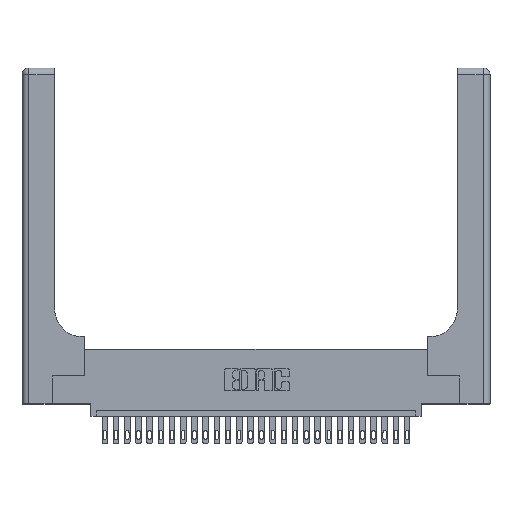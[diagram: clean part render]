
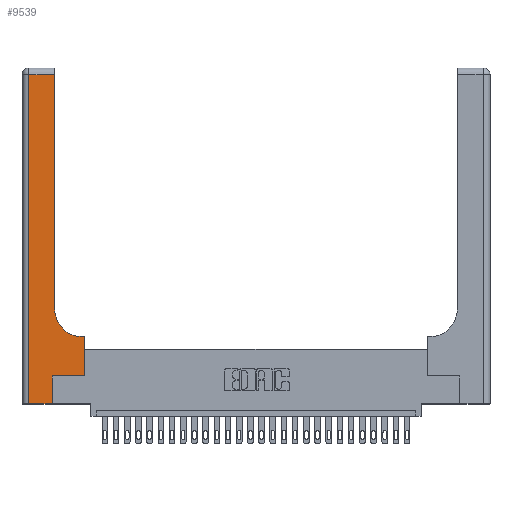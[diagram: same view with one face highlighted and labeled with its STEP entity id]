
A CAD part, top view. The second image highlights one B-rep face of the part: STEP entity #9539.
In plain terms, the highlighted planar face has unit normal (0, 0, 1).
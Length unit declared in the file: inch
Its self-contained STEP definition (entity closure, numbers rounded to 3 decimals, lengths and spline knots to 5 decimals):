
#55 = AXIS2_PLACEMENT_3D ( 'NONE', #7930, #12382, #5728 ) ;
#1465 = LINE ( 'NONE', #8245, #6556 ) ;
#1484 = EDGE_CURVE ( 'NONE', #8005, #10899, #6415, .T. ) ;
#1764 = DIRECTION ( 'NONE',  ( 0., -1., 0. ) ) ;
#2277 = DIRECTION ( 'NONE',  ( 0., 0., -1. ) ) ;
#3177 = DIRECTION ( 'NONE',  ( 0., 1., 0. ) ) ;
#3617 = EDGE_CURVE ( 'NONE', #11968, #6783, #13105, .T. ) ;
#3693 = DIRECTION ( 'NONE',  ( 0., 1., 0. ) ) ;
#3818 = DIRECTION ( 'NONE',  ( 1., 0., 0. ) ) ;
#4117 = EDGE_CURVE ( 'NONE', #6783, #14151, #5248, .T. ) ;
#4333 = VERTEX_POINT ( 'NONE', #11165 ) ;
#4653 = CARTESIAN_POINT ( 'NONE',  ( 0.269, 0., 0.37 ) ) ;
#5010 = EDGE_CURVE ( 'NONE', #26313, #11968, #1465, .T. ) ;
#5248 = LINE ( 'NONE', #4653, #22230 ) ;
#5728 = DIRECTION ( 'NONE',  ( -1., 0., 0. ) ) ;
#6003 = CARTESIAN_POINT ( 'NONE',  ( 0., 0., 0.37 ) ) ;
#6194 = EDGE_CURVE ( 'NONE', #14151, #4333, #14451, .T. ) ;
#6415 = CIRCLE ( 'NONE', #10715, 0.25 ) ;
#6529 = EDGE_CURVE ( 'NONE', #4333, #27735, #20626, .T. ) ;
#6556 = VECTOR ( 'NONE', #1764, 39.37008 ) ;
#6783 = VERTEX_POINT ( 'NONE', #25904 ) ;
#7451 = VECTOR ( 'NONE', #12882, 39.37008 ) ;
#7578 = CARTESIAN_POINT ( 'NONE',  ( 0.5585, 0.6, 0.37 ) ) ;
#7786 = EDGE_LOOP ( 'NONE', ( #13759, #9354, #21490, #13124, #13107, #12946, #10061, #17818, #15967 ) ) ;
#7930 = CARTESIAN_POINT ( 'NONE',  ( 0., 3., 0.37 ) ) ;
#8005 = VERTEX_POINT ( 'NONE', #16175 ) ;
#8196 = CARTESIAN_POINT ( 'NONE',  ( 0.269, 0.25, 0.37 ) ) ;
#8245 = CARTESIAN_POINT ( 'NONE',  ( 0.06, 3., 0.37 ) ) ;
#8307 = VECTOR ( 'NONE', #11509, 39.37008 ) ;
#9354 = ORIENTED_EDGE ( 'NONE', *, *, #20055, .T. ) ;
#9539 = ADVANCED_FACE ( 'NONE', ( #13238 ), #25222, .F. ) ;
#10061 = ORIENTED_EDGE ( 'NONE', *, *, #6529, .T. ) ;
#10715 = AXIS2_PLACEMENT_3D ( 'NONE', #15403, #2277, #15214 ) ;
#10899 = VERTEX_POINT ( 'NONE', #21075 ) ;
#11165 = CARTESIAN_POINT ( 'NONE',  ( 0.5585, 0.25, 0.37 ) ) ;
#11509 = DIRECTION ( 'NONE',  ( 1., 0., 0. ) ) ;
#11528 = CARTESIAN_POINT ( 'NONE',  ( 0.2915, 3., 0.37 ) ) ;
#11580 = DIRECTION ( 'NONE',  ( -1., 0., 0. ) ) ;
#11968 = VERTEX_POINT ( 'NONE', #14456 ) ;
#12089 = VECTOR ( 'NONE', #3818, 39.37008 ) ;
#12382 = DIRECTION ( 'NONE',  ( 0., 0., -1. ) ) ;
#12882 = DIRECTION ( 'NONE',  ( -1., 0., 0. ) ) ;
#12946 = ORIENTED_EDGE ( 'NONE', *, *, #6194, .T. ) ;
#13105 = LINE ( 'NONE', #6003, #12089 ) ;
#13107 = ORIENTED_EDGE ( 'NONE', *, *, #4117, .T. ) ;
#13124 = ORIENTED_EDGE ( 'NONE', *, *, #3617, .T. ) ;
#13238 = FACE_OUTER_BOUND ( 'NONE', #7786, .T. ) ;
#13477 = CARTESIAN_POINT ( 'NONE',  ( 0., 2.94, 0.37 ) ) ;
#13759 = ORIENTED_EDGE ( 'NONE', *, *, #26556, .T. ) ;
#14001 = EDGE_CURVE ( 'NONE', #27735, #8005, #19756, .T. ) ;
#14151 = VERTEX_POINT ( 'NONE', #8196 ) ;
#14451 = LINE ( 'NONE', #16187, #8307 ) ;
#14456 = CARTESIAN_POINT ( 'NONE',  ( 0.06, 0., 0.37 ) ) ;
#15214 = DIRECTION ( 'NONE',  ( 1., 0., 0. ) ) ;
#15403 = CARTESIAN_POINT ( 'NONE',  ( 0.5415, 0.85, 0.37 ) ) ;
#15719 = VERTEX_POINT ( 'NONE', #25510 ) ;
#15967 = ORIENTED_EDGE ( 'NONE', *, *, #1484, .T. ) ;
#16175 = CARTESIAN_POINT ( 'NONE',  ( 0.5415, 0.6, 0.37 ) ) ;
#16187 = CARTESIAN_POINT ( 'NONE',  ( 0.269, 0.25, 0.37 ) ) ;
#16505 = VECTOR ( 'NONE', #3693, 39.37008 ) ;
#16917 = CARTESIAN_POINT ( 'NONE',  ( 0.06, 2.94, 0.37 ) ) ;
#17684 = VECTOR ( 'NONE', #3177, 39.37008 ) ;
#17818 = ORIENTED_EDGE ( 'NONE', *, *, #14001, .T. ) ;
#18488 = VECTOR ( 'NONE', #11580, 39.37008 ) ;
#19756 = LINE ( 'NONE', #21746, #7451 ) ;
#20055 = EDGE_CURVE ( 'NONE', #15719, #26313, #24557, .T. ) ;
#20113 = DIRECTION ( 'NONE',  ( 0., 1., 0. ) ) ;
#20117 = LINE ( 'NONE', #11528, #17684 ) ;
#20626 = LINE ( 'NONE', #20741, #16505 ) ;
#20741 = CARTESIAN_POINT ( 'NONE',  ( 0.5585, 0.25, 0.37 ) ) ;
#21075 = CARTESIAN_POINT ( 'NONE',  ( 0.2915, 0.85, 0.37 ) ) ;
#21490 = ORIENTED_EDGE ( 'NONE', *, *, #5010, .T. ) ;
#21746 = CARTESIAN_POINT ( 'NONE',  ( 0.2915, 0.6, 0.37 ) ) ;
#22230 = VECTOR ( 'NONE', #20113, 39.37008 ) ;
#24557 = LINE ( 'NONE', #13477, #18488 ) ;
#25222 = PLANE ( 'NONE',  #55 ) ;
#25510 = CARTESIAN_POINT ( 'NONE',  ( 0.2915, 2.94, 0.37 ) ) ;
#25904 = CARTESIAN_POINT ( 'NONE',  ( 0.269, 0., 0.37 ) ) ;
#26313 = VERTEX_POINT ( 'NONE', #16917 ) ;
#26556 = EDGE_CURVE ( 'NONE', #10899, #15719, #20117, .T. ) ;
#27735 = VERTEX_POINT ( 'NONE', #7578 ) ;
